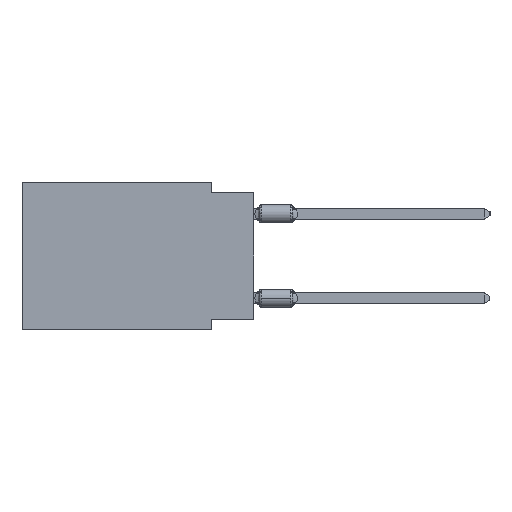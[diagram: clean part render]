
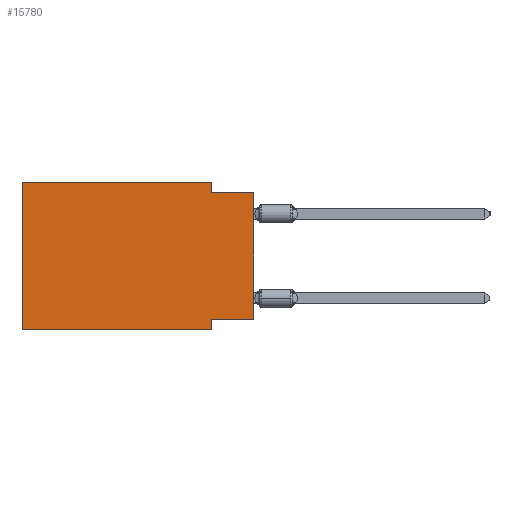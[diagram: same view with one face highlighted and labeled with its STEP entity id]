
A CAD part, left-side view. The second image highlights one B-rep face of the part: STEP entity #15780.
In plain terms, the highlighted planar face has unit normal (-1, 0, 0).
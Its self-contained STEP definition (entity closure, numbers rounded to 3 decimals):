
#31 = VERTEX_POINT ( 'NONE', #8531 ) ;
#227 = EDGE_CURVE ( 'NONE', #29689, #25924, #16159, .T. ) ;
#474 = LINE ( 'NONE', #9600, #40305 ) ;
#803 = DIRECTION ( 'NONE',  ( 0., 0., 1. ) ) ;
#1016 = CARTESIAN_POINT ( 'NONE',  ( 0., 2.54, -0.635 ) ) ;
#1347 = CARTESIAN_POINT ( 'NONE',  ( 0., 0., -0.635 ) ) ;
#1682 = EDGE_CURVE ( 'NONE', #33560, #31, #24694, .T. ) ;
#2063 = DIRECTION ( 'NONE',  ( 0., 0., 1. ) ) ;
#3811 = FACE_OUTER_BOUND ( 'NONE', #20549, .T. ) ;
#5344 = CARTESIAN_POINT ( 'NONE',  ( 0., 2.54, -8.89 ) ) ;
#6584 = VECTOR ( 'NONE', #2063, 1000. ) ;
#8531 = CARTESIAN_POINT ( 'NONE',  ( 0., 0., -0.635 ) ) ;
#8564 = DIRECTION ( 'NONE',  ( 0., 0., -1. ) ) ;
#8699 = EDGE_CURVE ( 'NONE', #25777, #26977, #474, .T. ) ;
#9039 = CARTESIAN_POINT ( 'NONE',  ( 0., 2.54, -8.255 ) ) ;
#9213 = CARTESIAN_POINT ( 'NONE',  ( 0., 13.97, -8.89 ) ) ;
#9600 = CARTESIAN_POINT ( 'NONE',  ( 0., 13.97, 0. ) ) ;
#10005 = CARTESIAN_POINT ( 'NONE',  ( 0., 13.97, -8.89 ) ) ;
#10367 = CARTESIAN_POINT ( 'NONE',  ( 0., 0., 0. ) ) ;
#10554 = DIRECTION ( 'NONE',  ( 0., 0., -1. ) ) ;
#13375 = DIRECTION ( 'NONE',  ( 0., 0., -1. ) ) ;
#13837 = VERTEX_POINT ( 'NONE', #9039 ) ;
#13944 = CARTESIAN_POINT ( 'NONE',  ( 0., 2.54, -8.89 ) ) ;
#14805 = EDGE_CURVE ( 'NONE', #34891, #31, #16940, .T. ) ;
#15780 = ADVANCED_FACE ( 'NONE', ( #3811 ), #16354, .F. ) ;
#16159 = LINE ( 'NONE', #10005, #20347 ) ;
#16354 = PLANE ( 'NONE',  #18127 ) ;
#16768 = CARTESIAN_POINT ( 'NONE',  ( 0., 13.97, 0. ) ) ;
#16940 = LINE ( 'NONE', #10367, #34459 ) ;
#17474 = CARTESIAN_POINT ( 'NONE',  ( 0., 2.54, 0. ) ) ;
#18127 = AXIS2_PLACEMENT_3D ( 'NONE', #16768, #39106, #13375 ) ;
#18476 = ORIENTED_EDGE ( 'NONE', *, *, #34608, .F. ) ;
#18610 = ORIENTED_EDGE ( 'NONE', *, *, #39684, .F. ) ;
#19963 = ORIENTED_EDGE ( 'NONE', *, *, #1682, .F. ) ;
#20106 = LINE ( 'NONE', #13944, #39566 ) ;
#20347 = VECTOR ( 'NONE', #22960, 1000. ) ;
#20417 = EDGE_CURVE ( 'NONE', #29689, #25777, #31173, .T. ) ;
#20490 = ORIENTED_EDGE ( 'NONE', *, *, #41550, .F. ) ;
#20549 = EDGE_LOOP ( 'NONE', ( #35979, #19963, #20490, #34499, #37635, #32319, #18610, #18476 ) ) ;
#20673 = DIRECTION ( 'NONE',  ( 0., -1., 0. ) ) ;
#21982 = VECTOR ( 'NONE', #8564, 1000. ) ;
#22743 = DIRECTION ( 'NONE',  ( 0., 1., 0. ) ) ;
#22776 = DIRECTION ( 'NONE',  ( 0., -1., 0. ) ) ;
#22960 = DIRECTION ( 'NONE',  ( 0., -1., 0. ) ) ;
#23162 = LINE ( 'NONE', #26366, #29457 ) ;
#24694 = LINE ( 'NONE', #1347, #36486 ) ;
#24719 = LINE ( 'NONE', #37698, #21982 ) ;
#25777 = VERTEX_POINT ( 'NONE', #33421 ) ;
#25924 = VERTEX_POINT ( 'NONE', #5344 ) ;
#26366 = CARTESIAN_POINT ( 'NONE',  ( 0., 0., -8.255 ) ) ;
#26977 = VERTEX_POINT ( 'NONE', #17474 ) ;
#28198 = CARTESIAN_POINT ( 'NONE',  ( 0., 13.97, 0. ) ) ;
#29457 = VECTOR ( 'NONE', #22743, 1000. ) ;
#29689 = VERTEX_POINT ( 'NONE', #9213 ) ;
#31173 = LINE ( 'NONE', #28198, #6584 ) ;
#32319 = ORIENTED_EDGE ( 'NONE', *, *, #227, .T. ) ;
#33357 = CARTESIAN_POINT ( 'NONE',  ( 0., 0., -8.255 ) ) ;
#33421 = CARTESIAN_POINT ( 'NONE',  ( 0., 13.97, 0. ) ) ;
#33560 = VERTEX_POINT ( 'NONE', #1016 ) ;
#34459 = VECTOR ( 'NONE', #803, 1000. ) ;
#34499 = ORIENTED_EDGE ( 'NONE', *, *, #8699, .F. ) ;
#34608 = EDGE_CURVE ( 'NONE', #34891, #13837, #23162, .T. ) ;
#34891 = VERTEX_POINT ( 'NONE', #33357 ) ;
#35979 = ORIENTED_EDGE ( 'NONE', *, *, #14805, .T. ) ;
#36486 = VECTOR ( 'NONE', #20673, 1000. ) ;
#37635 = ORIENTED_EDGE ( 'NONE', *, *, #20417, .F. ) ;
#37698 = CARTESIAN_POINT ( 'NONE',  ( 0., 2.54, 0. ) ) ;
#39106 = DIRECTION ( 'NONE',  ( 1., 0., 0. ) ) ;
#39566 = VECTOR ( 'NONE', #10554, 1000. ) ;
#39684 = EDGE_CURVE ( 'NONE', #13837, #25924, #20106, .T. ) ;
#40305 = VECTOR ( 'NONE', #22776, 1000. ) ;
#41550 = EDGE_CURVE ( 'NONE', #26977, #33560, #24719, .T. ) ;
